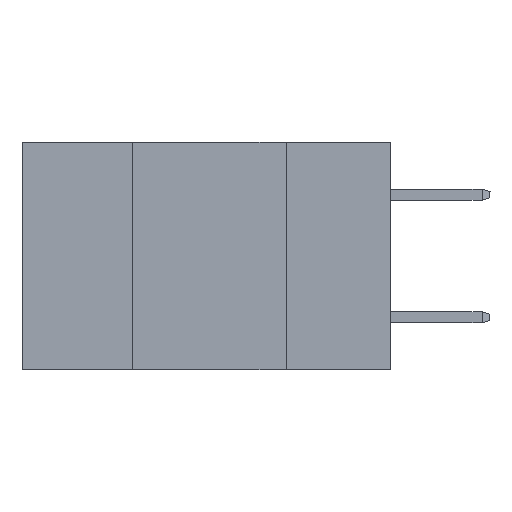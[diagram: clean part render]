
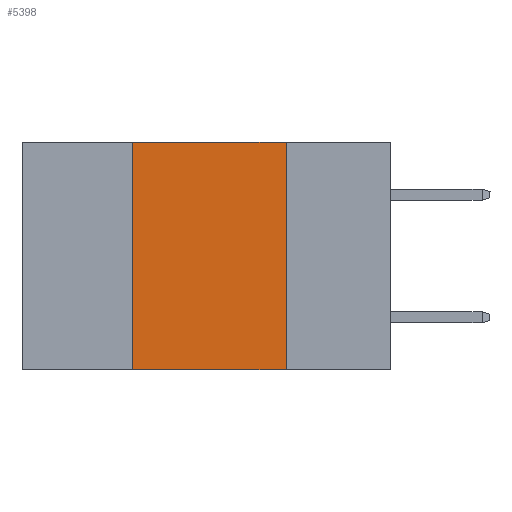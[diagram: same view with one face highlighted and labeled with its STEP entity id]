
A CAD part, left-side view. The second image highlights one B-rep face of the part: STEP entity #5398.
In plain terms, the highlighted planar face has unit normal (-1, 0, 0).
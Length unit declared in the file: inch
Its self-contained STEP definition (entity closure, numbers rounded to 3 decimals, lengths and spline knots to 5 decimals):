
#491 = CARTESIAN_POINT ( 'NONE',  ( 0., 0.6, -0.37 ) ) ;
#3282 = CARTESIAN_POINT ( 'NONE',  ( 0., 0.6, 0. ) ) ;
#3310 = CARTESIAN_POINT ( 'NONE',  ( 0., 0.6, 0. ) ) ;
#3516 = DIRECTION ( 'NONE',  ( 0., 0., -1. ) ) ;
#3534 = VERTEX_POINT ( 'NONE', #8751 ) ;
#4339 = LINE ( 'NONE', #5981, #14509 ) ;
#4963 = EDGE_CURVE ( 'NONE', #17588, #7857, #19407, .T. ) ;
#5002 = ORIENTED_EDGE ( 'NONE', *, *, #12175, .T. ) ;
#5398 = ADVANCED_FACE ( 'NONE', ( #6922 ), #21613, .F. ) ;
#5981 = CARTESIAN_POINT ( 'NONE',  ( 0., 0.17, 0. ) ) ;
#5985 = LINE ( 'NONE', #491, #12649 ) ;
#6420 = CARTESIAN_POINT ( 'NONE',  ( 0., 0.42, 0. ) ) ;
#6922 = FACE_OUTER_BOUND ( 'NONE', #19326, .T. ) ;
#7289 = CARTESIAN_POINT ( 'NONE',  ( 0., 0.42, -0.37 ) ) ;
#7857 = VERTEX_POINT ( 'NONE', #11460 ) ;
#8367 = AXIS2_PLACEMENT_3D ( 'NONE', #3282, #8702, #3516 ) ;
#8702 = DIRECTION ( 'NONE',  ( 1., 0., 0. ) ) ;
#8751 = CARTESIAN_POINT ( 'NONE',  ( 0., 0.17, -0.37 ) ) ;
#9652 = EDGE_CURVE ( 'NONE', #17453, #17588, #9834, .T. ) ;
#9834 = LINE ( 'NONE', #6420, #22778 ) ;
#10494 = DIRECTION ( 'NONE',  ( 0., -1., 0. ) ) ;
#11460 = CARTESIAN_POINT ( 'NONE',  ( 0., 0.17, 0. ) ) ;
#12175 = EDGE_CURVE ( 'NONE', #17453, #3534, #5985, .T. ) ;
#12649 = VECTOR ( 'NONE', #20230, 39.37008 ) ;
#13754 = ORIENTED_EDGE ( 'NONE', *, *, #4963, .F. ) ;
#14509 = VECTOR ( 'NONE', #22100, 39.37008 ) ;
#14914 = CARTESIAN_POINT ( 'NONE',  ( 0., 0.42, 0. ) ) ;
#17006 = DIRECTION ( 'NONE',  ( 0., 0., 1. ) ) ;
#17453 = VERTEX_POINT ( 'NONE', #7289 ) ;
#17491 = EDGE_CURVE ( 'NONE', #7857, #3534, #4339, .T. ) ;
#17588 = VERTEX_POINT ( 'NONE', #14914 ) ;
#19326 = EDGE_LOOP ( 'NONE', ( #19862, #13754, #22390, #5002 ) ) ;
#19407 = LINE ( 'NONE', #3310, #20744 ) ;
#19862 = ORIENTED_EDGE ( 'NONE', *, *, #17491, .F. ) ;
#20230 = DIRECTION ( 'NONE',  ( 0., -1., 0. ) ) ;
#20744 = VECTOR ( 'NONE', #10494, 39.37008 ) ;
#21613 = PLANE ( 'NONE',  #8367 ) ;
#22100 = DIRECTION ( 'NONE',  ( 0., 0., -1. ) ) ;
#22390 = ORIENTED_EDGE ( 'NONE', *, *, #9652, .F. ) ;
#22778 = VECTOR ( 'NONE', #17006, 39.37008 ) ;
